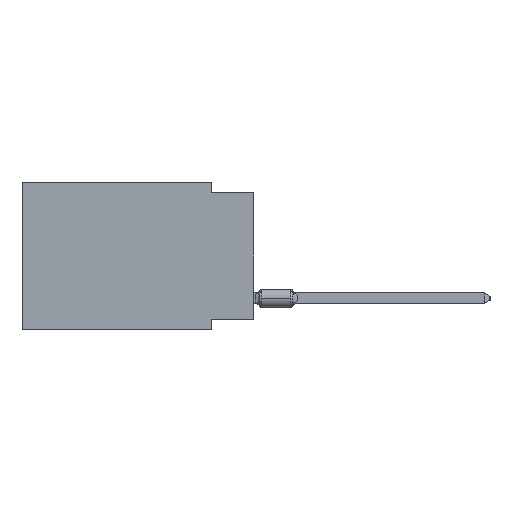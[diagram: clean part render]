
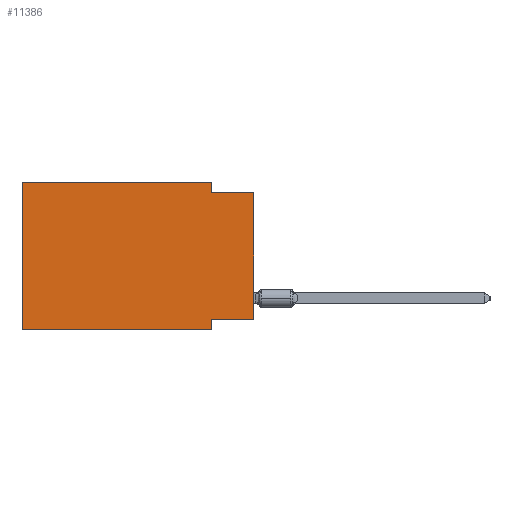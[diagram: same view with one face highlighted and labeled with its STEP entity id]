
A CAD part, left-side view. The second image highlights one B-rep face of the part: STEP entity #11386.
In plain terms, the highlighted planar face has unit normal (-1, 0, 0).
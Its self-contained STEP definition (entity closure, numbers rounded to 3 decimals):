
#711 = VERTEX_POINT ( 'NONE', #37234 ) ;
#1800 = CARTESIAN_POINT ( 'NONE',  ( 0., 13.97, 0. ) ) ;
#4820 = EDGE_CURVE ( 'NONE', #711, #18213, #7936, .T. ) ;
#5758 = CARTESIAN_POINT ( 'NONE',  ( 0., 0., -8.255 ) ) ;
#7918 = LINE ( 'NONE', #59106, #69445 ) ;
#7936 = LINE ( 'NONE', #13800, #53394 ) ;
#8537 = PLANE ( 'NONE',  #38062 ) ;
#8759 = EDGE_CURVE ( 'NONE', #11393, #50325, #51653, .T. ) ;
#8772 = EDGE_LOOP ( 'NONE', ( #74252, #38259, #61368, #68691, #27865, #81284, #55329, #64157 ) ) ;
#9767 = DIRECTION ( 'NONE',  ( 0., 0., -1. ) ) ;
#10177 = DIRECTION ( 'NONE',  ( 1., 0., 0. ) ) ;
#11386 = ADVANCED_FACE ( 'NONE', ( #65989 ), #8537, .F. ) ;
#11393 = VERTEX_POINT ( 'NONE', #23590 ) ;
#12386 = EDGE_CURVE ( 'NONE', #711, #20684, #30524, .T. ) ;
#13800 = CARTESIAN_POINT ( 'NONE',  ( 0., 0., 0. ) ) ;
#14510 = EDGE_CURVE ( 'NONE', #35108, #65586, #25752, .T. ) ;
#14939 = EDGE_CURVE ( 'NONE', #65586, #18213, #81480, .T. ) ;
#15130 = DIRECTION ( 'NONE',  ( 0., 0., 1. ) ) ;
#16684 = CARTESIAN_POINT ( 'NONE',  ( 0., 13.97, -8.89 ) ) ;
#16719 = EDGE_CURVE ( 'NONE', #50325, #35108, #7918, .T. ) ;
#18213 = VERTEX_POINT ( 'NONE', #81700 ) ;
#18332 = DIRECTION ( 'NONE',  ( 0., 1., 0. ) ) ;
#20684 = VERTEX_POINT ( 'NONE', #51122 ) ;
#22216 = EDGE_CURVE ( 'NONE', #11393, #80241, #48152, .T. ) ;
#23590 = CARTESIAN_POINT ( 'NONE',  ( 0., 13.97, -8.89 ) ) ;
#25752 = LINE ( 'NONE', #30791, #65134 ) ;
#27865 = ORIENTED_EDGE ( 'NONE', *, *, #8759, .F. ) ;
#30524 = LINE ( 'NONE', #5758, #66456 ) ;
#30791 = CARTESIAN_POINT ( 'NONE',  ( 0., 2.54, 0. ) ) ;
#35108 = VERTEX_POINT ( 'NONE', #48328 ) ;
#36391 = VECTOR ( 'NONE', #15130, 1000. ) ;
#37110 = VECTOR ( 'NONE', #68886, 1000. ) ;
#37234 = CARTESIAN_POINT ( 'NONE',  ( 0., 0., -8.255 ) ) ;
#38062 = AXIS2_PLACEMENT_3D ( 'NONE', #53422, #10177, #9767 ) ;
#38259 = ORIENTED_EDGE ( 'NONE', *, *, #14939, .F. ) ;
#38318 = DIRECTION ( 'NONE',  ( 0., 0., -1. ) ) ;
#40658 = CARTESIAN_POINT ( 'NONE',  ( 0., 2.54, -0.635 ) ) ;
#42057 = CARTESIAN_POINT ( 'NONE',  ( 0., 2.54, -8.89 ) ) ;
#45262 = DIRECTION ( 'NONE',  ( 0., -1., 0. ) ) ;
#48152 = LINE ( 'NONE', #16684, #67856 ) ;
#48328 = CARTESIAN_POINT ( 'NONE',  ( 0., 2.54, 0. ) ) ;
#50325 = VERTEX_POINT ( 'NONE', #1800 ) ;
#51122 = CARTESIAN_POINT ( 'NONE',  ( 0., 2.54, -8.255 ) ) ;
#51653 = LINE ( 'NONE', #72616, #36391 ) ;
#53394 = VECTOR ( 'NONE', #64144, 1000. ) ;
#53422 = CARTESIAN_POINT ( 'NONE',  ( 0., 13.97, 0. ) ) ;
#54038 = DIRECTION ( 'NONE',  ( 0., -1., 0. ) ) ;
#54405 = LINE ( 'NONE', #54831, #57939 ) ;
#54831 = CARTESIAN_POINT ( 'NONE',  ( 0., 2.54, -8.89 ) ) ;
#55329 = ORIENTED_EDGE ( 'NONE', *, *, #56815, .F. ) ;
#56815 = EDGE_CURVE ( 'NONE', #20684, #80241, #54405, .T. ) ;
#57939 = VECTOR ( 'NONE', #67400, 1000. ) ;
#59106 = CARTESIAN_POINT ( 'NONE',  ( 0., 13.97, 0. ) ) ;
#61368 = ORIENTED_EDGE ( 'NONE', *, *, #14510, .F. ) ;
#64144 = DIRECTION ( 'NONE',  ( 0., 0., 1. ) ) ;
#64157 = ORIENTED_EDGE ( 'NONE', *, *, #12386, .F. ) ;
#65134 = VECTOR ( 'NONE', #38318, 1000. ) ;
#65586 = VERTEX_POINT ( 'NONE', #40658 ) ;
#65989 = FACE_OUTER_BOUND ( 'NONE', #8772, .T. ) ;
#66456 = VECTOR ( 'NONE', #18332, 1000. ) ;
#67400 = DIRECTION ( 'NONE',  ( 0., 0., -1. ) ) ;
#67856 = VECTOR ( 'NONE', #54038, 1000. ) ;
#68691 = ORIENTED_EDGE ( 'NONE', *, *, #16719, .F. ) ;
#68886 = DIRECTION ( 'NONE',  ( 0., -1., 0. ) ) ;
#69445 = VECTOR ( 'NONE', #45262, 1000. ) ;
#72616 = CARTESIAN_POINT ( 'NONE',  ( 0., 13.97, 0. ) ) ;
#74252 = ORIENTED_EDGE ( 'NONE', *, *, #4820, .T. ) ;
#76005 = CARTESIAN_POINT ( 'NONE',  ( 0., 0., -0.635 ) ) ;
#80241 = VERTEX_POINT ( 'NONE', #42057 ) ;
#81284 = ORIENTED_EDGE ( 'NONE', *, *, #22216, .T. ) ;
#81480 = LINE ( 'NONE', #76005, #37110 ) ;
#81700 = CARTESIAN_POINT ( 'NONE',  ( 0., 0., -0.635 ) ) ;
